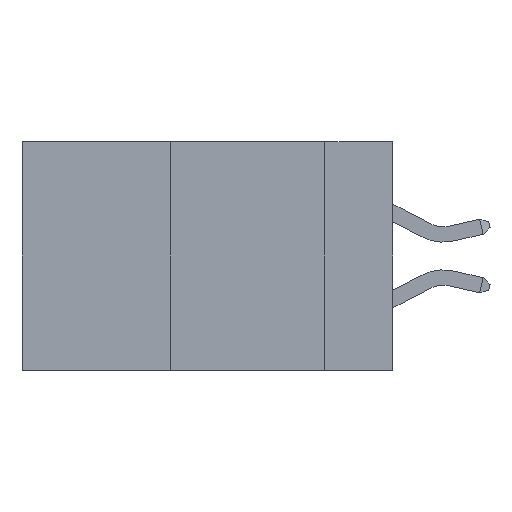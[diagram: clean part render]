
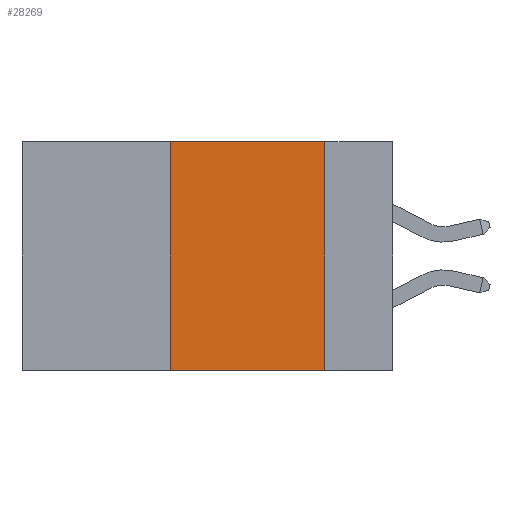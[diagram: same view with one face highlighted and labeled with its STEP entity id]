
A CAD part, left-side view. The second image highlights one B-rep face of the part: STEP entity #28269.
In plain terms, the highlighted planar face has unit normal (-1, 0, 0).
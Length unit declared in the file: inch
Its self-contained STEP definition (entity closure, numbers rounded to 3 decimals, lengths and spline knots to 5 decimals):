
#2508 = VERTEX_POINT ( 'NONE', #39033 ) ;
#2648 = VECTOR ( 'NONE', #35770, 39.37008 ) ;
#3678 = CARTESIAN_POINT ( 'NONE',  ( 0., 0.11, 0. ) ) ;
#3736 = PLANE ( 'NONE',  #17172 ) ;
#4604 = VERTEX_POINT ( 'NONE', #7220 ) ;
#5067 = EDGE_CURVE ( 'NONE', #2508, #41971, #35547, .T. ) ;
#7054 = DIRECTION ( 'NONE',  ( 0., 0., -1. ) ) ;
#7126 = ORIENTED_EDGE ( 'NONE', *, *, #19228, .F. ) ;
#7220 = CARTESIAN_POINT ( 'NONE',  ( 0., 0.36, 0. ) ) ;
#9604 = VECTOR ( 'NONE', #40063, 39.37008 ) ;
#10908 = CARTESIAN_POINT ( 'NONE',  ( 0., 0.36, 0. ) ) ;
#11332 = VECTOR ( 'NONE', #30630, 39.37008 ) ;
#12812 = CARTESIAN_POINT ( 'NONE',  ( 0., 0.6, -0.37 ) ) ;
#14003 = CARTESIAN_POINT ( 'NONE',  ( 0., 0.11, 0. ) ) ;
#17172 = AXIS2_PLACEMENT_3D ( 'NONE', #20200, #39752, #7054 ) ;
#19108 = LINE ( 'NONE', #10908, #11332 ) ;
#19228 = EDGE_CURVE ( 'NONE', #23670, #41971, #25458, .T. ) ;
#20200 = CARTESIAN_POINT ( 'NONE',  ( 0., 0.6, 0. ) ) ;
#20691 = CARTESIAN_POINT ( 'NONE',  ( 0., 0.11, -0.37 ) ) ;
#22993 = FACE_OUTER_BOUND ( 'NONE', #30850, .T. ) ;
#23670 = VERTEX_POINT ( 'NONE', #3678 ) ;
#24973 = EDGE_CURVE ( 'NONE', #2508, #4604, #19108, .T. ) ;
#25458 = LINE ( 'NONE', #14003, #34169 ) ;
#26696 = ORIENTED_EDGE ( 'NONE', *, *, #24973, .F. ) ;
#28269 = ADVANCED_FACE ( 'NONE', ( #22993 ), #3736, .F. ) ;
#30630 = DIRECTION ( 'NONE',  ( 0., 0., 1. ) ) ;
#30850 = EDGE_LOOP ( 'NONE', ( #7126, #32339, #26696, #39103 ) ) ;
#32339 = ORIENTED_EDGE ( 'NONE', *, *, #32907, .F. ) ;
#32907 = EDGE_CURVE ( 'NONE', #4604, #23670, #35808, .T. ) ;
#33663 = DIRECTION ( 'NONE',  ( 0., 0., -1. ) ) ;
#34169 = VECTOR ( 'NONE', #33663, 39.37008 ) ;
#35547 = LINE ( 'NONE', #12812, #2648 ) ;
#35770 = DIRECTION ( 'NONE',  ( 0., -1., 0. ) ) ;
#35808 = LINE ( 'NONE', #36793, #9604 ) ;
#36793 = CARTESIAN_POINT ( 'NONE',  ( 0., 0.6, 0. ) ) ;
#39033 = CARTESIAN_POINT ( 'NONE',  ( 0., 0.36, -0.37 ) ) ;
#39103 = ORIENTED_EDGE ( 'NONE', *, *, #5067, .T. ) ;
#39752 = DIRECTION ( 'NONE',  ( 1., 0., 0. ) ) ;
#40063 = DIRECTION ( 'NONE',  ( 0., -1., 0. ) ) ;
#41971 = VERTEX_POINT ( 'NONE', #20691 ) ;
